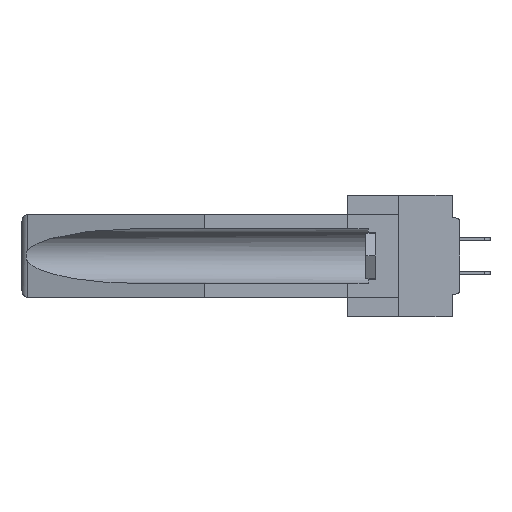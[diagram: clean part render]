
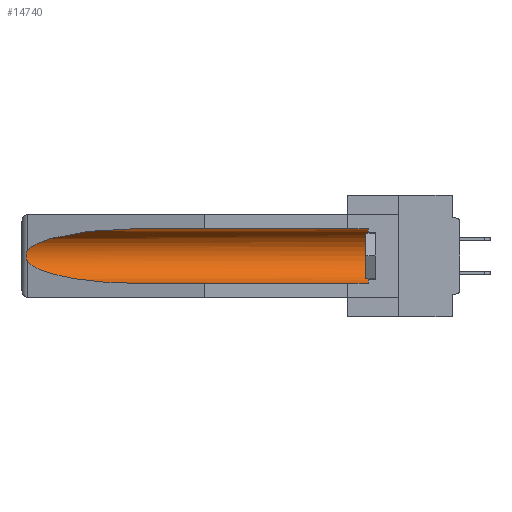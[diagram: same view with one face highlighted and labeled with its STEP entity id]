
A CAD part, left-side view. The second image highlights one B-rep face of the part: STEP entity #14740.
In plain terms, the highlighted cylindrical face has radius 2.857 mm (diameter 5.715 mm), a partial arc.
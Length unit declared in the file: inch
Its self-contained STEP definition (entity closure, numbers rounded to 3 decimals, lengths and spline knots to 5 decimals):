
#561 = CARTESIAN_POINT ( 'NONE',  ( 0.26537, 1.52718, -0.19328 ) ) ;
#1874 = EDGE_CURVE ( 'NONE', #29672, #26828, #18002, .T. ) ;
#1880 = AXIS2_PLACEMENT_3D ( 'NONE', #24261, #27127, #18895 ) ;
#2152 = EDGE_CURVE ( 'NONE', #26828, #20412, #33510, .T. ) ;
#2185 = CARTESIAN_POINT ( 'NONE',  ( 0.2675, 1.53308, -0.17534 ) ) ;
#2294 = CARTESIAN_POINT ( 'NONE',  ( 0.26597, 1.52961, -0.15275 ) ) ;
#2421 = CARTESIAN_POINT ( 'NONE',  ( 0.2673, 1.5327, -0.16383 ) ) ;
#2916 = DIRECTION ( 'NONE',  ( 0., 0., 1. ) ) ;
#3302 = DIRECTION ( 'NONE',  ( 0., 1., 0. ) ) ;
#3417 = CARTESIAN_POINT ( 'NONE',  ( 0.155, -0.30754, -0.059 ) ) ;
#3597 = CARTESIAN_POINT ( 'NONE',  ( 0.26537, 1.52718, -0.14972 ) ) ;
#4161 = FACE_OUTER_BOUND ( 'NONE', #11531, .T. ) ;
#5186 = CARTESIAN_POINT ( 'NONE',  ( 0.26537, 1.52718, -0.19328 ) ) ;
#5793 = DIRECTION ( 'NONE',  ( 0., 1., 0. ) ) ;
#6819 = CARTESIAN_POINT ( 'NONE',  ( 0.155, 0.126, -0.059 ) ) ;
#7390 = CARTESIAN_POINT ( 'NONE',  ( 0.25451, 1.48313, -0.24835 ) ) ;
#7509 = CARTESIAN_POINT ( 'NONE',  ( 0.155, 1.07973, -0.284 ) ) ;
#8237 = VERTEX_POINT ( 'NONE', #21391 ) ;
#8577 = CARTESIAN_POINT ( 'NONE',  ( 0.155, 0.126, -0.1715 ) ) ;
#10259 = VERTEX_POINT ( 'NONE', #6819 ) ;
#10531 = CARTESIAN_POINT ( 'NONE',  ( 0.2675, 1.53308, -0.16763 ) ) ;
#11531 = EDGE_LOOP ( 'NONE', ( #12850, #13428, #28819, #29190, #18922, #14652 ) ) ;
#12281 =( BOUNDED_CURVE ( )  B_SPLINE_CURVE ( 3, ( #13263, #7390, #23782, #7509 ),
 .UNSPECIFIED., .F., .F. ) 
 B_SPLINE_CURVE_WITH_KNOTS ( ( 4, 4 ),
 ( 0.1948, 1.5708 ),
 .UNSPECIFIED. ) 
 CURVE ( )  GEOMETRIC_REPRESENTATION_ITEM ( )  RATIONAL_B_SPLINE_CURVE ( ( 1., 0.848, 0.848, 1. ) ) 
 REPRESENTATION_ITEM ( '' )  );
#12850 = ORIENTED_EDGE ( 'NONE', *, *, #1874, .T. ) ;
#13064 = LINE ( 'NONE', #24827, #32309 ) ;
#13263 = CARTESIAN_POINT ( 'NONE',  ( 0.26537, 1.52718, -0.19328 ) ) ;
#13428 = ORIENTED_EDGE ( 'NONE', *, *, #2152, .T. ) ;
#14442 = CARTESIAN_POINT ( 'NONE',  ( 0.155, 1.07973, -0.059 ) ) ;
#14643 = EDGE_CURVE ( 'NONE', #20412, #19522, #12281, .T. ) ;
#14652 = ORIENTED_EDGE ( 'NONE', *, *, #32970, .T. ) ;
#14740 = ADVANCED_FACE ( 'NONE', ( #4161 ), #25052, .F. ) ;
#15612 = CARTESIAN_POINT ( 'NONE',  ( 0.2673, 1.53269, -0.17917 ) ) ;
#15723 = EDGE_CURVE ( 'NONE', #8237, #19522, #13064, .T. ) ;
#16002 = CARTESIAN_POINT ( 'NONE',  ( 0.25451, 1.48313, -0.09465 ) ) ;
#18002 =( BOUNDED_CURVE ( )  B_SPLINE_CURVE ( 3, ( #29674, #23672, #16002, #26795 ),
 .UNSPECIFIED., .F., .F. ) 
 B_SPLINE_CURVE_WITH_KNOTS ( ( 4, 4 ),
 ( 4.71239, 6.08839 ),
 .UNSPECIFIED. ) 
 CURVE ( )  GEOMETRIC_REPRESENTATION_ITEM ( )  RATIONAL_B_SPLINE_CURVE ( ( 1., 0.848, 0.848, 1. ) ) 
 REPRESENTATION_ITEM ( '' )  );
#18756 = CARTESIAN_POINT ( 'NONE',  ( 0.26654, 1.53092, -0.15636 ) ) ;
#18895 = DIRECTION ( 'NONE',  ( 0., 0., 1. ) ) ;
#18922 = ORIENTED_EDGE ( 'NONE', *, *, #20173, .T. ) ;
#19263 = VECTOR ( 'NONE', #3302, 39.37008 ) ;
#19397 = AXIS2_PLACEMENT_3D ( 'NONE', #8577, #24511, #2916 ) ;
#19522 = VERTEX_POINT ( 'NONE', #24686 ) ;
#20173 = EDGE_CURVE ( 'NONE', #8237, #10259, #32816, .T. ) ;
#20412 = VERTEX_POINT ( 'NONE', #561 ) ;
#21391 = CARTESIAN_POINT ( 'NONE',  ( 0.155, 0.126, -0.284 ) ) ;
#21478 = CARTESIAN_POINT ( 'NONE',  ( 0.26597, 1.5296, -0.19026 ) ) ;
#23672 = CARTESIAN_POINT ( 'NONE',  ( 0.21114, 1.30732, -0.059 ) ) ;
#23782 = CARTESIAN_POINT ( 'NONE',  ( 0.21114, 1.30732, -0.284 ) ) ;
#23880 = CARTESIAN_POINT ( 'NONE',  ( 0.26537, 1.52718, -0.14972 ) ) ;
#24261 = CARTESIAN_POINT ( 'NONE',  ( 0.155, -0.30754, -0.1715 ) ) ;
#24511 = DIRECTION ( 'NONE',  ( 0., -1., 0. ) ) ;
#24686 = CARTESIAN_POINT ( 'NONE',  ( 0.155, 1.07973, -0.284 ) ) ;
#24827 = CARTESIAN_POINT ( 'NONE',  ( 0.155, -0.30754, -0.284 ) ) ;
#25052 = CYLINDRICAL_SURFACE ( 'NONE', #1880, 0.1125 ) ;
#26543 = LINE ( 'NONE', #3417, #19263 ) ;
#26795 = CARTESIAN_POINT ( 'NONE',  ( 0.26537, 1.52718, -0.14972 ) ) ;
#26828 = VERTEX_POINT ( 'NONE', #3597 ) ;
#27127 = DIRECTION ( 'NONE',  ( 0., 1., 0. ) ) ;
#28819 = ORIENTED_EDGE ( 'NONE', *, *, #14643, .T. ) ;
#29190 = ORIENTED_EDGE ( 'NONE', *, *, #15723, .F. ) ;
#29672 = VERTEX_POINT ( 'NONE', #14442 ) ;
#29674 = CARTESIAN_POINT ( 'NONE',  ( 0.155, 1.07973, -0.059 ) ) ;
#32309 = VECTOR ( 'NONE', #5793, 39.37008 ) ;
#32483 = CARTESIAN_POINT ( 'NONE',  ( 0.26655, 1.53094, -0.18657 ) ) ;
#32816 = CIRCLE ( 'NONE', #19397, 0.1125 ) ;
#32970 = EDGE_CURVE ( 'NONE', #10259, #29672, #26543, .T. ) ;
#33510 = B_SPLINE_CURVE_WITH_KNOTS ( 'NONE', 3,
 ( #23880, #2294, #18756, #2421, #10531, #2185, #15612, #32483, #21478, #5186 ),
 .UNSPECIFIED., .F., .F.,
 ( 4, 2, 2, 2, 4 ),
 ( 0., 0.00029, 0.00058, 0.00087, 0.00117 ),
 .UNSPECIFIED. ) ;
